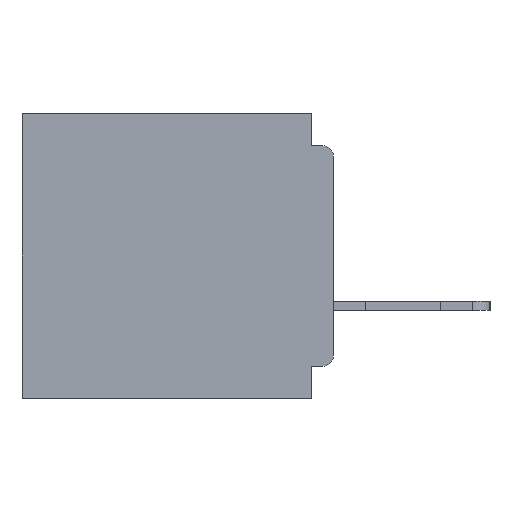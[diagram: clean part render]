
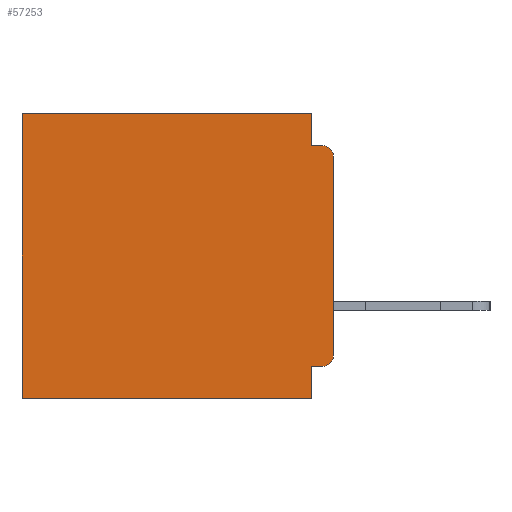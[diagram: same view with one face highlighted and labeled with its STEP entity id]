
A CAD part, left-side view. The second image highlights one B-rep face of the part: STEP entity #57253.
In plain terms, the highlighted planar face has unit normal (-1, 0, 0).
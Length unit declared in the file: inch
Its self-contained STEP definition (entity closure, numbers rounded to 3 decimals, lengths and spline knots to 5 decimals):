
#912 = AXIS2_PLACEMENT_3D ( 'NONE', #61867, #33110, #3850 ) ;
#1764 = EDGE_CURVE ( 'NONE', #2328, #29822, #38954, .T. ) ;
#1977 = EDGE_CURVE ( 'NONE', #10892, #32290, #54738, .T. ) ;
#2328 = VERTEX_POINT ( 'NONE', #22258 ) ;
#2610 = CARTESIAN_POINT ( 'NONE',  ( 0.3, 0.031, 0. ) ) ;
#3141 = DIRECTION ( 'NONE',  ( 0., -1., 0. ) ) ;
#3464 = CARTESIAN_POINT ( 'NONE',  ( 0.3, 0.015, -0.045 ) ) ;
#3850 = DIRECTION ( 'NONE',  ( 0., 0., -1. ) ) ;
#5537 = CIRCLE ( 'NONE', #16981, 0.015 ) ;
#8964 = ORIENTED_EDGE ( 'NONE', *, *, #48252, .F. ) ;
#8991 = VECTOR ( 'NONE', #57047, 39.37008 ) ;
#10001 = EDGE_LOOP ( 'NONE', ( #8964, #22127, #24158, #53361, #21199, #27857, #17960, #39766, #34012, #53796 ) ) ;
#10892 = VERTEX_POINT ( 'NONE', #27287 ) ;
#11721 = VERTEX_POINT ( 'NONE', #3464 ) ;
#12835 = DIRECTION ( 'NONE',  ( 0., 0., -1. ) ) ;
#12976 = VECTOR ( 'NONE', #12835, 39.37008 ) ;
#13409 = PLANE ( 'NONE',  #912 ) ;
#15319 = EDGE_CURVE ( 'NONE', #31501, #59730, #5537, .T. ) ;
#15839 = CARTESIAN_POINT ( 'NONE',  ( 0.3, 0.437, -0.4 ) ) ;
#16637 = CARTESIAN_POINT ( 'NONE',  ( 0.3, 0.015, -0.34 ) ) ;
#16826 = CARTESIAN_POINT ( 'NONE',  ( 0.3, 0.031, 0. ) ) ;
#16981 = AXIS2_PLACEMENT_3D ( 'NONE', #16637, #50654, #21585 ) ;
#17960 = ORIENTED_EDGE ( 'NONE', *, *, #18113, .F. ) ;
#18113 = EDGE_CURVE ( 'NONE', #32290, #29822, #48321, .T. ) ;
#19574 = DIRECTION ( 'NONE',  ( 0., 0., -1. ) ) ;
#19905 = DIRECTION ( 'NONE',  ( 0., 0., -1. ) ) ;
#20198 = VERTEX_POINT ( 'NONE', #47001 ) ;
#20543 = LINE ( 'NONE', #16826, #44882 ) ;
#21199 = ORIENTED_EDGE ( 'NONE', *, *, #37324, .T. ) ;
#21585 = DIRECTION ( 'NONE',  ( 0., 0., -1. ) ) ;
#22127 = ORIENTED_EDGE ( 'NONE', *, *, #60913, .T. ) ;
#22258 = CARTESIAN_POINT ( 'NONE',  ( 0.3, 0.437, 0. ) ) ;
#22288 = VERTEX_POINT ( 'NONE', #25223 ) ;
#22345 = CARTESIAN_POINT ( 'NONE',  ( 0.3, 0.015, -0.06 ) ) ;
#24158 = ORIENTED_EDGE ( 'NONE', *, *, #26366, .F. ) ;
#24523 = CARTESIAN_POINT ( 'NONE',  ( 0.3, 0., -0.34 ) ) ;
#25223 = CARTESIAN_POINT ( 'NONE',  ( 0.3, 0., -0.06 ) ) ;
#25563 = CARTESIAN_POINT ( 'NONE',  ( 0.3, 0., -0.355 ) ) ;
#26366 = EDGE_CURVE ( 'NONE', #20198, #11721, #60296, .T. ) ;
#27281 = DIRECTION ( 'NONE',  ( 0., 0., -1. ) ) ;
#27287 = CARTESIAN_POINT ( 'NONE',  ( 0.3, 0.031, -0.355 ) ) ;
#27857 = ORIENTED_EDGE ( 'NONE', *, *, #1764, .T. ) ;
#29822 = VERTEX_POINT ( 'NONE', #15839 ) ;
#29975 = DIRECTION ( 'NONE',  ( 0., 1., 0. ) ) ;
#30435 = DIRECTION ( 'NONE',  ( 0., 1., 0. ) ) ;
#31501 = VERTEX_POINT ( 'NONE', #52985 ) ;
#32290 = VERTEX_POINT ( 'NONE', #55492 ) ;
#33110 = DIRECTION ( 'NONE',  ( 1., 0., 0. ) ) ;
#33525 = VECTOR ( 'NONE', #19574, 39.37008 ) ;
#34012 = ORIENTED_EDGE ( 'NONE', *, *, #34067, .F. ) ;
#34067 = EDGE_CURVE ( 'NONE', #31501, #10892, #49813, .T. ) ;
#36271 = VECTOR ( 'NONE', #3141, 39.37008 ) ;
#36296 = EDGE_CURVE ( 'NONE', #44067, #20198, #20543, .T. ) ;
#36504 = LINE ( 'NONE', #52040, #8991 ) ;
#36999 = VECTOR ( 'NONE', #29975, 39.37008 ) ;
#37324 = EDGE_CURVE ( 'NONE', #44067, #2328, #36504, .T. ) ;
#38954 = LINE ( 'NONE', #41097, #12976 ) ;
#39766 = ORIENTED_EDGE ( 'NONE', *, *, #1977, .F. ) ;
#41097 = CARTESIAN_POINT ( 'NONE',  ( 0.3, 0.437, -0.4 ) ) ;
#41920 = VECTOR ( 'NONE', #19905, 39.37008 ) ;
#43843 = CARTESIAN_POINT ( 'NONE',  ( 0.3, 0., -0.4 ) ) ;
#44067 = VERTEX_POINT ( 'NONE', #2610 ) ;
#44882 = VECTOR ( 'NONE', #60393, 39.37008 ) ;
#46371 = LINE ( 'NONE', #43843, #33525 ) ;
#46981 = CARTESIAN_POINT ( 'NONE',  ( 0.3, 0., -0.045 ) ) ;
#47001 = CARTESIAN_POINT ( 'NONE',  ( 0.3, 0.031, -0.045 ) ) ;
#48252 = EDGE_CURVE ( 'NONE', #22288, #59730, #46371, .T. ) ;
#48270 = VECTOR ( 'NONE', #30435, 39.37008 ) ;
#48321 = LINE ( 'NONE', #58800, #36999 ) ;
#49394 = CIRCLE ( 'NONE', #51515, 0.015 ) ;
#49813 = LINE ( 'NONE', #25563, #48270 ) ;
#50654 = DIRECTION ( 'NONE',  ( -1., 0., 0. ) ) ;
#51515 = AXIS2_PLACEMENT_3D ( 'NONE', #22345, #56177, #27281 ) ;
#52040 = CARTESIAN_POINT ( 'NONE',  ( 0.3, 0., 0. ) ) ;
#52985 = CARTESIAN_POINT ( 'NONE',  ( 0.3, 0.015, -0.355 ) ) ;
#53361 = ORIENTED_EDGE ( 'NONE', *, *, #36296, .F. ) ;
#53796 = ORIENTED_EDGE ( 'NONE', *, *, #15319, .T. ) ;
#54738 = LINE ( 'NONE', #58201, #41920 ) ;
#55492 = CARTESIAN_POINT ( 'NONE',  ( 0.3, 0.031, -0.4 ) ) ;
#56080 = FACE_OUTER_BOUND ( 'NONE', #10001, .T. ) ;
#56177 = DIRECTION ( 'NONE',  ( -1., 0., 0. ) ) ;
#57047 = DIRECTION ( 'NONE',  ( 0., 1., 0. ) ) ;
#57253 = ADVANCED_FACE ( 'NONE', ( #56080 ), #13409, .F. ) ;
#58201 = CARTESIAN_POINT ( 'NONE',  ( 0.3, 0.031, -0.4 ) ) ;
#58800 = CARTESIAN_POINT ( 'NONE',  ( 0.3, 0., -0.4 ) ) ;
#59730 = VERTEX_POINT ( 'NONE', #24523 ) ;
#60296 = LINE ( 'NONE', #46981, #36271 ) ;
#60393 = DIRECTION ( 'NONE',  ( 0., 0., -1. ) ) ;
#60913 = EDGE_CURVE ( 'NONE', #22288, #11721, #49394, .T. ) ;
#61867 = CARTESIAN_POINT ( 'NONE',  ( 0.3, 0., -0.4 ) ) ;
